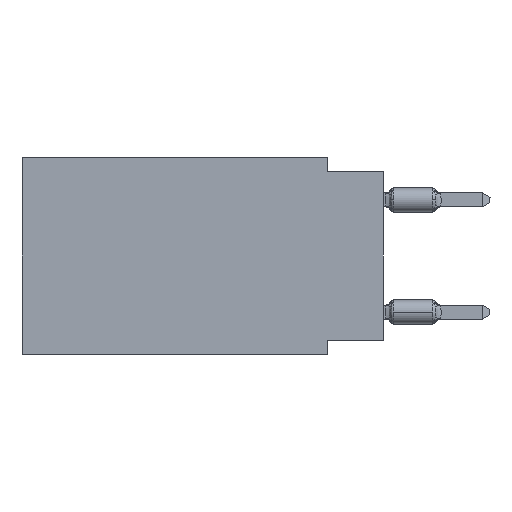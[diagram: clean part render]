
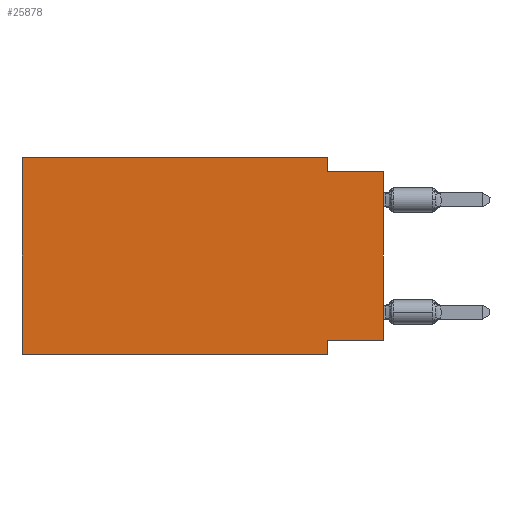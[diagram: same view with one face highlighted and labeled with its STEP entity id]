
A CAD part, left-side view. The second image highlights one B-rep face of the part: STEP entity #25878.
In plain terms, the highlighted planar face has unit normal (-1, 0, 0).
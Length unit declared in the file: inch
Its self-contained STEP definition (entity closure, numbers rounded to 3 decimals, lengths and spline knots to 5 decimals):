
#459 = LINE ( 'NONE', #15886, #12569 ) ;
#503 = CARTESIAN_POINT ( 'NONE',  ( 0., 0.645, 0. ) ) ;
#1618 = VERTEX_POINT ( 'NONE', #39519 ) ;
#2781 = DIRECTION ( 'NONE',  ( 1., 0., 0. ) ) ;
#2842 = EDGE_CURVE ( 'NONE', #16181, #20955, #35801, .T. ) ;
#3133 = CARTESIAN_POINT ( 'NONE',  ( 0., 0.645, -0.35 ) ) ;
#3849 = ORIENTED_EDGE ( 'NONE', *, *, #14601, .F. ) ;
#4282 = VECTOR ( 'NONE', #31570, 39.37008 ) ;
#4504 = CARTESIAN_POINT ( 'NONE',  ( 0., 0.645, 0. ) ) ;
#5492 = VERTEX_POINT ( 'NONE', #18518 ) ;
#5761 = DIRECTION ( 'NONE',  ( 0., 0., 1. ) ) ;
#6330 = FACE_OUTER_BOUND ( 'NONE', #22185, .T. ) ;
#6799 = VECTOR ( 'NONE', #5761, 39.37008 ) ;
#9373 = ORIENTED_EDGE ( 'NONE', *, *, #35524, .T. ) ;
#9793 = VECTOR ( 'NONE', #19655, 39.37008 ) ;
#10324 = LINE ( 'NONE', #29516, #33931 ) ;
#10790 = LINE ( 'NONE', #30730, #22455 ) ;
#10962 = LINE ( 'NONE', #3133, #46129 ) ;
#11414 = ORIENTED_EDGE ( 'NONE', *, *, #23850, .F. ) ;
#11577 = DIRECTION ( 'NONE',  ( 0., -1., 0. ) ) ;
#11791 = LINE ( 'NONE', #42364, #16574 ) ;
#12569 = VECTOR ( 'NONE', #11577, 39.37008 ) ;
#13512 = VERTEX_POINT ( 'NONE', #33440 ) ;
#13609 = CARTESIAN_POINT ( 'NONE',  ( 0., 0., 0. ) ) ;
#14601 = EDGE_CURVE ( 'NONE', #24563, #5492, #459, .T. ) ;
#15886 = CARTESIAN_POINT ( 'NONE',  ( 0., 0., -0.025 ) ) ;
#16181 = VERTEX_POINT ( 'NONE', #503 ) ;
#16574 = VECTOR ( 'NONE', #49685, 39.37008 ) ;
#16679 = LINE ( 'NONE', #20715, #4282 ) ;
#17562 = ORIENTED_EDGE ( 'NONE', *, *, #2842, .F. ) ;
#17713 = PLANE ( 'NONE',  #24439 ) ;
#17925 = EDGE_CURVE ( 'NONE', #36733, #35062, #16679, .T. ) ;
#18192 = DIRECTION ( 'NONE',  ( 0., 0., -1. ) ) ;
#18518 = CARTESIAN_POINT ( 'NONE',  ( 0., 0., -0.025 ) ) ;
#19655 = DIRECTION ( 'NONE',  ( 0., -1., 0. ) ) ;
#20715 = CARTESIAN_POINT ( 'NONE',  ( 0., 0., -0.325 ) ) ;
#20729 = ORIENTED_EDGE ( 'NONE', *, *, #17925, .F. ) ;
#20955 = VERTEX_POINT ( 'NONE', #44833 ) ;
#22185 = EDGE_LOOP ( 'NONE', ( #29397, #3849, #11414, #17562, #41477, #9373, #33071, #20729 ) ) ;
#22455 = VECTOR ( 'NONE', #46441, 39.37008 ) ;
#23850 = EDGE_CURVE ( 'NONE', #20955, #24563, #10324, .T. ) ;
#24439 = AXIS2_PLACEMENT_3D ( 'NONE', #28828, #2781, #18192 ) ;
#24563 = VERTEX_POINT ( 'NONE', #48604 ) ;
#25878 = ADVANCED_FACE ( 'NONE', ( #6330 ), #17713, .F. ) ;
#28828 = CARTESIAN_POINT ( 'NONE',  ( 0., 0.645, 0. ) ) ;
#29397 = ORIENTED_EDGE ( 'NONE', *, *, #37106, .T. ) ;
#29516 = CARTESIAN_POINT ( 'NONE',  ( 0., 0.1, 0. ) ) ;
#30500 = EDGE_CURVE ( 'NONE', #1618, #16181, #10790, .T. ) ;
#30730 = CARTESIAN_POINT ( 'NONE',  ( 0., 0.645, 0. ) ) ;
#31570 = DIRECTION ( 'NONE',  ( 0., 1., 0. ) ) ;
#32858 = CARTESIAN_POINT ( 'NONE',  ( 0., 0., -0.325 ) ) ;
#33071 = ORIENTED_EDGE ( 'NONE', *, *, #45703, .F. ) ;
#33440 = CARTESIAN_POINT ( 'NONE',  ( 0., 0.1, -0.35 ) ) ;
#33931 = VECTOR ( 'NONE', #48979, 39.37008 ) ;
#35062 = VERTEX_POINT ( 'NONE', #48462 ) ;
#35524 = EDGE_CURVE ( 'NONE', #1618, #13512, #10962, .T. ) ;
#35801 = LINE ( 'NONE', #4504, #9793 ) ;
#36733 = VERTEX_POINT ( 'NONE', #32858 ) ;
#37106 = EDGE_CURVE ( 'NONE', #36733, #5492, #40622, .T. ) ;
#39519 = CARTESIAN_POINT ( 'NONE',  ( 0., 0.645, -0.35 ) ) ;
#40622 = LINE ( 'NONE', #13609, #6799 ) ;
#41477 = ORIENTED_EDGE ( 'NONE', *, *, #30500, .F. ) ;
#42024 = DIRECTION ( 'NONE',  ( 0., -1., 0. ) ) ;
#42364 = CARTESIAN_POINT ( 'NONE',  ( 0., 0.1, -0.35 ) ) ;
#44833 = CARTESIAN_POINT ( 'NONE',  ( 0., 0.1, 0. ) ) ;
#45703 = EDGE_CURVE ( 'NONE', #35062, #13512, #11791, .T. ) ;
#46129 = VECTOR ( 'NONE', #42024, 39.37008 ) ;
#46441 = DIRECTION ( 'NONE',  ( 0., 0., 1. ) ) ;
#48462 = CARTESIAN_POINT ( 'NONE',  ( 0., 0.1, -0.325 ) ) ;
#48604 = CARTESIAN_POINT ( 'NONE',  ( 0., 0.1, -0.025 ) ) ;
#48979 = DIRECTION ( 'NONE',  ( 0., 0., -1. ) ) ;
#49685 = DIRECTION ( 'NONE',  ( 0., 0., -1. ) ) ;
